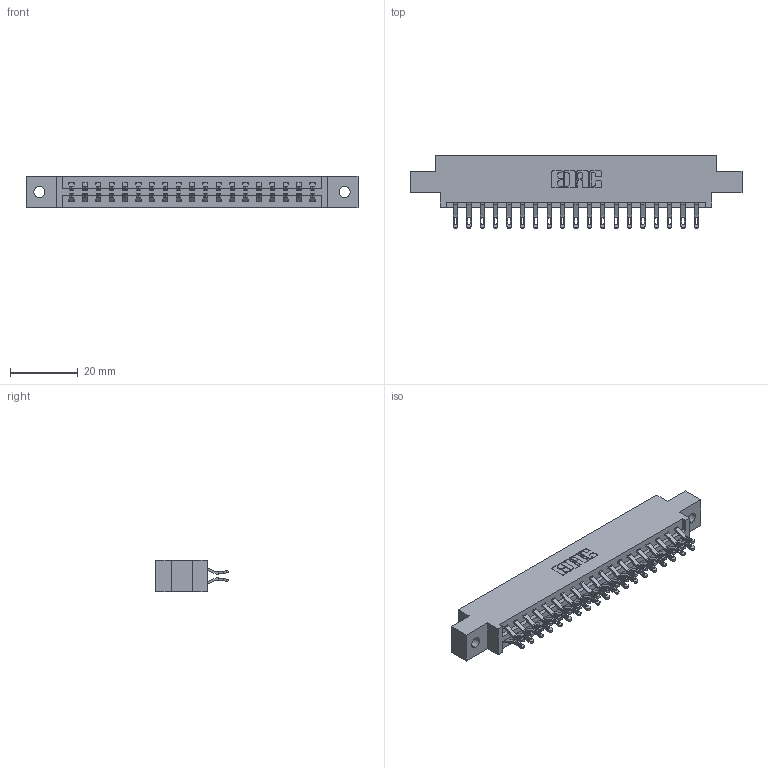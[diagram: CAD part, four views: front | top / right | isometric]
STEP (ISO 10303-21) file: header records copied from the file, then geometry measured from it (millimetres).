
FILE_DESCRIPTION (( 'STEP AP203' ), '1' );
FILE_NAME ('337-038-555-802.STEP', '2019-10-11T11:31:32', ( '' ), ( '' ), 'SwSTEP 2.0', 'SolidWorks 2016', '' );
FILE_SCHEMA (( 'CONFIG_CONTROL_DESIGN' ));
Length unit declared in the file: inch
Products named in the file (3): 337-038-555-802; 345-292-001_555 Tail; 337 Part_0.170 Offset - 0.128 Dia
Assembly tree (39 placements, depth 2):
  337-038-555-802
    337 Part_0.170 Offset - 0.128 Dia
    345-292-001_555 Tail  x38
Bounding box: 98.3 x 21.47 x 9.4 mm (x, y, z)
Volume: 10009.3 mm3; surface area: 11342.6 mm2
Topology: 39 solids, 39 shells, 2398 faces, 7505 edges, 5002 vertices
Faces by surface type: plane 1442, cylinder 956
Entity records: 18167 total; most frequent: CARTESIAN_POINT 3116, ORIENTED_EDGE 3022, DIRECTION 2663, EDGE_CURVE 1511, LINE 1363, VECTOR 1363, VERTEX_POINT 1006, AXIS2_PLACEMENT_3D 650
